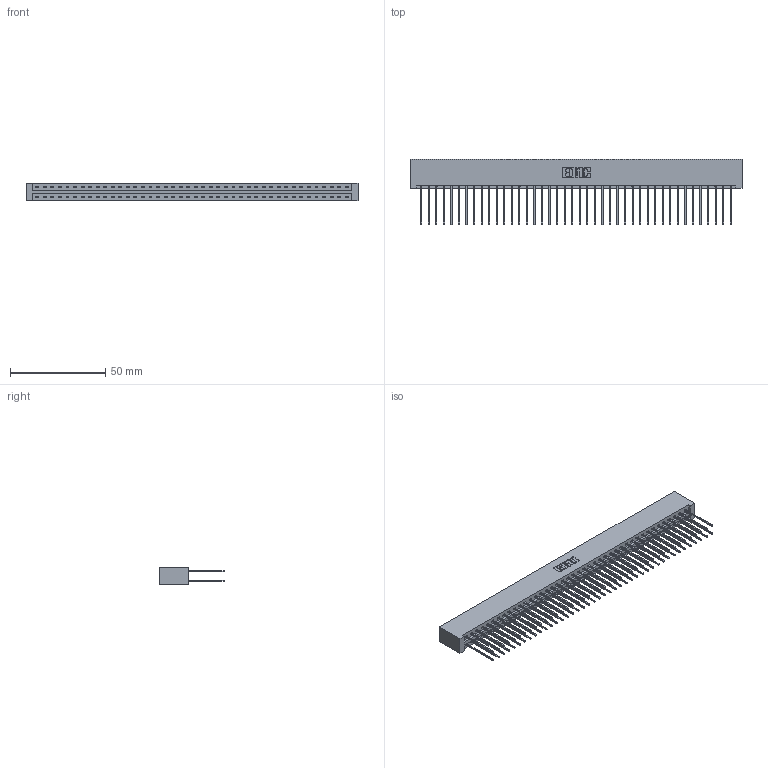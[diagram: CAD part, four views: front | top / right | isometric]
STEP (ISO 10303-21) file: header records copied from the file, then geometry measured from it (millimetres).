
FILE_DESCRIPTION (( 'STEP AP203' ), '1' );
FILE_NAME ('387-084-541-201.STEP', '2019-10-23T01:27:42', ( '' ), ( '' ), 'SwSTEP 2.0', 'SolidWorks 2016', '' );
FILE_SCHEMA (( 'CONFIG_CONTROL_DESIGN' ));
Length unit declared in the file: inch
Products named in the file (3): 337 Part_No Mounting Lugs; 387-084-541-201; 345-292-001_345-293-141
Assembly tree (85 placements, depth 2):
  387-084-541-201
    337 Part_No Mounting Lugs
    345-292-001_345-293-141  x84
Bounding box: 174.29 x 34.3 x 9.4 mm (x, y, z)
Volume: 19611.2 mm3; surface area: 24645.6 mm2
Topology: 85 solids, 85 shells, 4642 faces, 13811 edges, 9094 vertices
Faces by surface type: plane 3258, cylinder 1384
Entity records: 32305 total; most frequent: CARTESIAN_POINT 5442, ORIENTED_EDGE 5378, DIRECTION 4621, EDGE_CURVE 2689, LINE 2569, VECTOR 2569, VERTEX_POINT 1790, AXIS2_PLACEMENT_3D 1026
